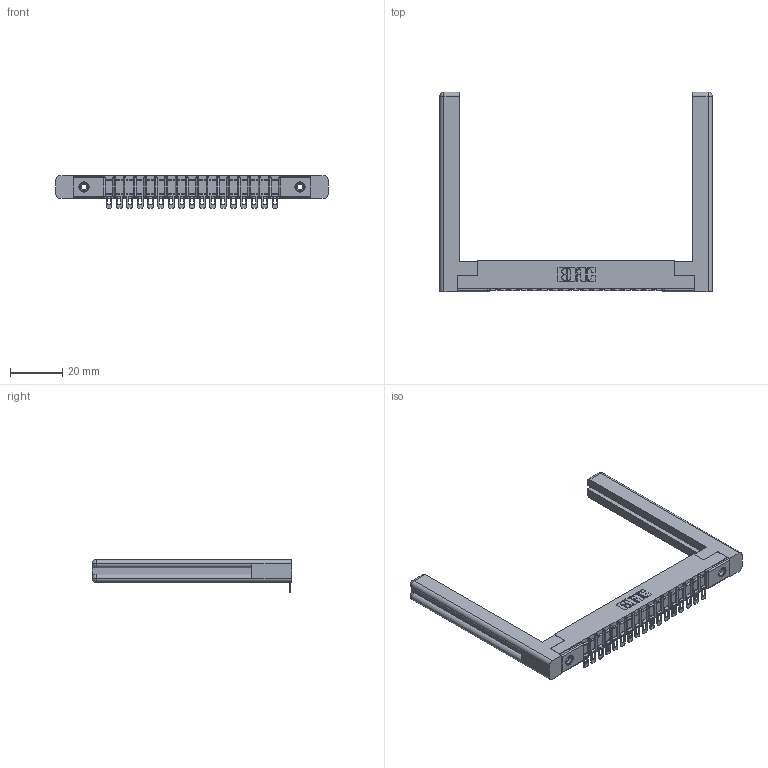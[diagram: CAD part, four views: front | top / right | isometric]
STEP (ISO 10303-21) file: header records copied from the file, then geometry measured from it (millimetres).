
FILE_DESCRIPTION (( 'STEP AP203' ), '1' );
FILE_NAME ('357-017-454-158.STEP', '2020-09-30T23:05:23', ( '' ), ( '' ), 'SwSTEP 2.0', 'SolidWorks 2020', '' );
FILE_SCHEMA (( 'CONFIG_CONTROL_DESIGN' ));
Length unit declared in the file: inch
Products named in the file (5): 307-220-058; 357-017-454-158; 307-290-002_554; 345-250-001_345-250-001-102; 307 Part_.156 Dia Mounting Holes
Assembly tree (22 placements, depth 2):
  357-017-454-158
    307 Part_.156 Dia Mounting Holes
    307-290-002_554  x17
    307-220-058  x2
    345-250-001_345-250-001-102  x2
Bounding box: 103.99 x 76.33 x 12.52 mm (x, y, z)
Volume: 14546.9 mm3; surface area: 17309 mm2
Topology: 22 solids, 22 shells, 1655 faces, 4978 edges, 3256 vertices
Faces by surface type: plane 936, cylinder 659, sphere 36, torus 12, cone 12
Entity records: 21254 total; most frequent: CARTESIAN_POINT 3589, ORIENTED_EDGE 3518, DIRECTION 3465, EDGE_CURVE 1759, VECTOR 1325, LINE 1325, VERTEX_POINT 1140, AXIS2_PLACEMENT_3D 1070
